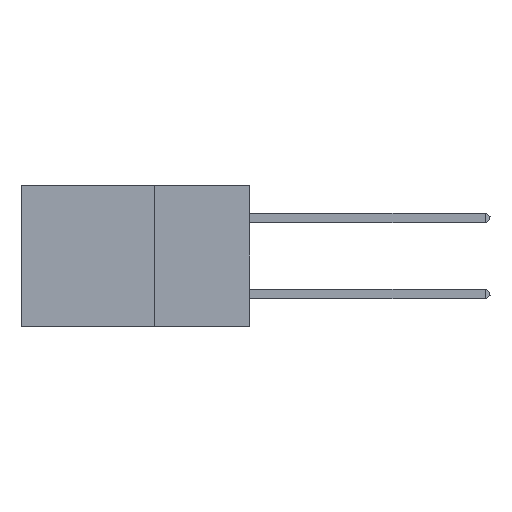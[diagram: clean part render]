
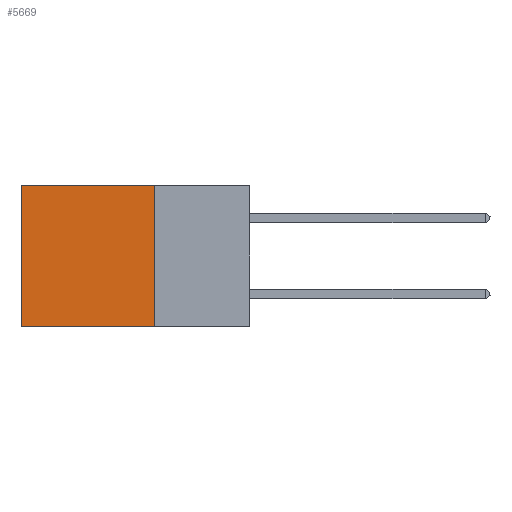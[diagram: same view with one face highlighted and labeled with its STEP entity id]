
A CAD part, left-side view. The second image highlights one B-rep face of the part: STEP entity #5669.
In plain terms, the highlighted planar face has unit normal (-1, 0, 0).
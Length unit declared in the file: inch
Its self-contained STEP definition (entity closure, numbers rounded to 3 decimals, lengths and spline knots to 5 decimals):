
#1197 = DIRECTION ( 'NONE',  ( 0., 0., -1. ) ) ;
#4535 = ORIENTED_EDGE ( 'NONE', *, *, #41224, .F. ) ;
#4790 = CARTESIAN_POINT ( 'NONE',  ( 0.2875, 0.25, 0. ) ) ;
#4923 = PLANE ( 'NONE',  #8835 ) ;
#5669 = ADVANCED_FACE ( 'NONE', ( #37214 ), #4923, .F. ) ;
#8835 = AXIS2_PLACEMENT_3D ( 'NONE', #4790, #25262, #1197 ) ;
#10021 = CARTESIAN_POINT ( 'NONE',  ( 0.2875, 0.25, 0. ) ) ;
#10590 = CARTESIAN_POINT ( 'NONE',  ( 0.2875, 0.6, 0. ) ) ;
#10834 = ORIENTED_EDGE ( 'NONE', *, *, #40059, .T. ) ;
#11014 = VECTOR ( 'NONE', #12845, 39.37008 ) ;
#12366 = ORIENTED_EDGE ( 'NONE', *, *, #29645, .T. ) ;
#12479 = VERTEX_POINT ( 'NONE', #27999 ) ;
#12845 = DIRECTION ( 'NONE',  ( 0., 1., 0. ) ) ;
#13143 = LINE ( 'NONE', #10021, #11014 ) ;
#14953 = EDGE_LOOP ( 'NONE', ( #10834, #36908, #4535, #12366 ) ) ;
#15014 = CARTESIAN_POINT ( 'NONE',  ( 0.2875, 0.25, 0. ) ) ;
#15687 = VERTEX_POINT ( 'NONE', #15014 ) ;
#19119 = VECTOR ( 'NONE', #37573, 39.37008 ) ;
#20257 = VECTOR ( 'NONE', #26537, 39.37008 ) ;
#23792 = CARTESIAN_POINT ( 'NONE',  ( 0.2875, 0.25, -0.37 ) ) ;
#24553 = LINE ( 'NONE', #41346, #19119 ) ;
#24687 = VECTOR ( 'NONE', #27728, 39.37008 ) ;
#25110 = LINE ( 'NONE', #32901, #20257 ) ;
#25262 = DIRECTION ( 'NONE',  ( 1., 0., 0. ) ) ;
#26537 = DIRECTION ( 'NONE',  ( 0., 1., 0. ) ) ;
#27519 = CARTESIAN_POINT ( 'NONE',  ( 0.2875, 0.6, -0.37 ) ) ;
#27728 = DIRECTION ( 'NONE',  ( 0., 0., -1. ) ) ;
#27842 = EDGE_CURVE ( 'NONE', #32204, #36316, #25110, .T. ) ;
#27999 = CARTESIAN_POINT ( 'NONE',  ( 0.2875, 0.6, 0. ) ) ;
#29645 = EDGE_CURVE ( 'NONE', #15687, #12479, #13143, .T. ) ;
#32204 = VERTEX_POINT ( 'NONE', #23792 ) ;
#32901 = CARTESIAN_POINT ( 'NONE',  ( 0.2875, 0.25, -0.37 ) ) ;
#33864 = LINE ( 'NONE', #10590, #24687 ) ;
#36316 = VERTEX_POINT ( 'NONE', #27519 ) ;
#36908 = ORIENTED_EDGE ( 'NONE', *, *, #27842, .F. ) ;
#37214 = FACE_OUTER_BOUND ( 'NONE', #14953, .T. ) ;
#37573 = DIRECTION ( 'NONE',  ( 0., 0., -1. ) ) ;
#40059 = EDGE_CURVE ( 'NONE', #12479, #36316, #33864, .T. ) ;
#41224 = EDGE_CURVE ( 'NONE', #15687, #32204, #24553, .T. ) ;
#41346 = CARTESIAN_POINT ( 'NONE',  ( 0.2875, 0.25, 0. ) ) ;
